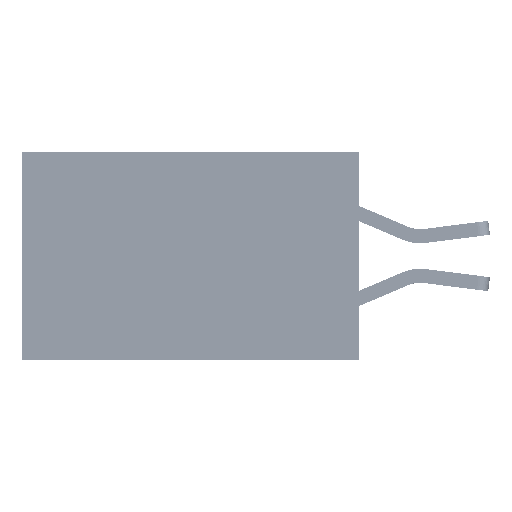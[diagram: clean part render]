
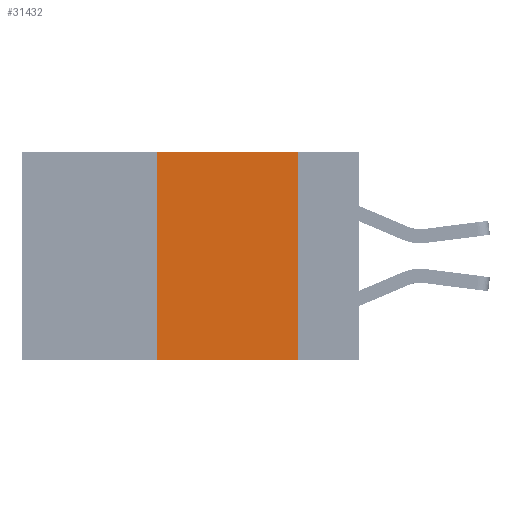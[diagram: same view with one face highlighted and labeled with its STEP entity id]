
A CAD part, left-side view. The second image highlights one B-rep face of the part: STEP entity #31432.
In plain terms, the highlighted planar face has unit normal (-1, 0, 0).
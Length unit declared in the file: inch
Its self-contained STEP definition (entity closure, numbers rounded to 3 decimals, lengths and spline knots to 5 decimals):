
#1031 = DIRECTION ( 'NONE',  ( 0., -1., 0. ) ) ;
#1504 = ORIENTED_EDGE ( 'NONE', *, *, #5162, .F. ) ;
#2008 = VECTOR ( 'NONE', #1031, 39.37008 ) ;
#2066 = CARTESIAN_POINT ( 'NONE',  ( 0., 0.11, -0.37 ) ) ;
#3230 = CARTESIAN_POINT ( 'NONE',  ( 0., 0.6, 0. ) ) ;
#4866 = VERTEX_POINT ( 'NONE', #16911 ) ;
#5162 = EDGE_CURVE ( 'NONE', #16416, #18736, #30610, .T. ) ;
#6058 = LINE ( 'NONE', #21687, #19165 ) ;
#7284 = DIRECTION ( 'NONE',  ( 0., 0., 1. ) ) ;
#8446 = DIRECTION ( 'NONE',  ( 0., 0., -1. ) ) ;
#9873 = PLANE ( 'NONE',  #10321 ) ;
#10321 = AXIS2_PLACEMENT_3D ( 'NONE', #3230, #38436, #19598 ) ;
#10561 = ORIENTED_EDGE ( 'NONE', *, *, #28724, .T. ) ;
#14068 = VERTEX_POINT ( 'NONE', #2066 ) ;
#16416 = VERTEX_POINT ( 'NONE', #29474 ) ;
#16911 = CARTESIAN_POINT ( 'NONE',  ( 0., 0.11, 0. ) ) ;
#17004 = CARTESIAN_POINT ( 'NONE',  ( 0., 0.36, 0. ) ) ;
#17050 = LINE ( 'NONE', #33906, #24524 ) ;
#17860 = EDGE_CURVE ( 'NONE', #4866, #14068, #17050, .T. ) ;
#18685 = ORIENTED_EDGE ( 'NONE', *, *, #27681, .F. ) ;
#18736 = VERTEX_POINT ( 'NONE', #22738 ) ;
#19165 = VECTOR ( 'NONE', #24868, 39.37008 ) ;
#19598 = DIRECTION ( 'NONE',  ( 0., 0., -1. ) ) ;
#20178 = LINE ( 'NONE', #20361, #2008 ) ;
#20361 = CARTESIAN_POINT ( 'NONE',  ( 0., 0.6, -0.37 ) ) ;
#20694 = ORIENTED_EDGE ( 'NONE', *, *, #17860, .F. ) ;
#21450 = EDGE_LOOP ( 'NONE', ( #20694, #18685, #1504, #10561 ) ) ;
#21687 = CARTESIAN_POINT ( 'NONE',  ( 0., 0.6, 0. ) ) ;
#22738 = CARTESIAN_POINT ( 'NONE',  ( 0., 0.36, 0. ) ) ;
#24524 = VECTOR ( 'NONE', #8446, 39.37008 ) ;
#24868 = DIRECTION ( 'NONE',  ( 0., -1., 0. ) ) ;
#27681 = EDGE_CURVE ( 'NONE', #18736, #4866, #6058, .T. ) ;
#28724 = EDGE_CURVE ( 'NONE', #16416, #14068, #20178, .T. ) ;
#29474 = CARTESIAN_POINT ( 'NONE',  ( 0., 0.36, -0.37 ) ) ;
#30610 = LINE ( 'NONE', #17004, #37982 ) ;
#31432 = ADVANCED_FACE ( 'NONE', ( #34758 ), #9873, .F. ) ;
#33906 = CARTESIAN_POINT ( 'NONE',  ( 0., 0.11, 0. ) ) ;
#34758 = FACE_OUTER_BOUND ( 'NONE', #21450, .T. ) ;
#37982 = VECTOR ( 'NONE', #7284, 39.37008 ) ;
#38436 = DIRECTION ( 'NONE',  ( 1., 0., 0. ) ) ;
